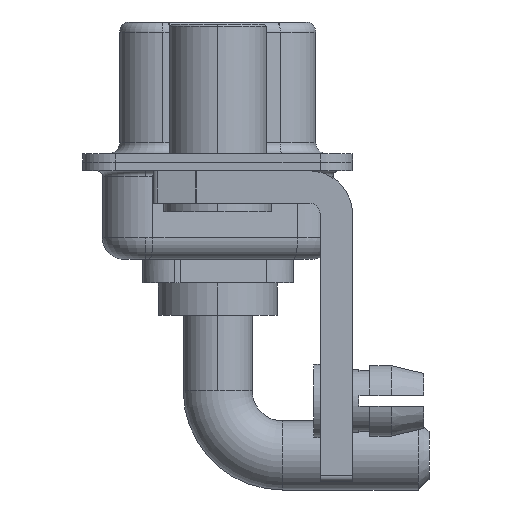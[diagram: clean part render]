
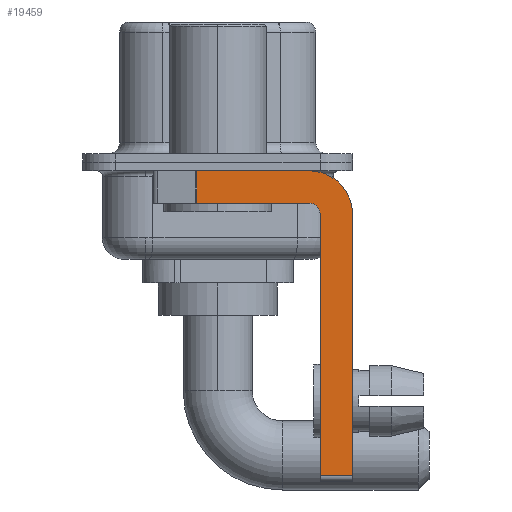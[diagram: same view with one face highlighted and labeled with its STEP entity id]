
A CAD part, left-side view. The second image highlights one B-rep face of the part: STEP entity #19459.
In plain terms, the highlighted planar face has unit normal (-1, 0, 0).
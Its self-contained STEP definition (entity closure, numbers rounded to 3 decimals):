
#223 = VERTEX_POINT ( 'NONE', #592 ) ;
#592 = CARTESIAN_POINT ( 'NONE',  ( -2.9, -6.25, -14.55 ) ) ;
#1279 = CARTESIAN_POINT ( 'NONE',  ( -2.9, -4.25, -14.55 ) ) ;
#1299 = VECTOR ( 'NONE', #8342, 1000. ) ;
#1378 = ORIENTED_EDGE ( 'NONE', *, *, #16896, .F. ) ;
#1668 = VERTEX_POINT ( 'NONE', #7297 ) ;
#1797 = CIRCLE ( 'NONE', #13898, 0.5 ) ;
#2083 = LINE ( 'NONE', #5151, #1299 ) ;
#2265 = CIRCLE ( 'NONE', #13045, 2. ) ;
#2371 = CARTESIAN_POINT ( 'NONE',  ( -2.9, -4.75, -14.8 ) ) ;
#2719 = VERTEX_POINT ( 'NONE', #2897 ) ;
#2897 = CARTESIAN_POINT ( 'NONE',  ( -2.9, -4.75, -2.4 ) ) ;
#2933 = EDGE_CURVE ( 'NONE', #13169, #2719, #6983, .T. ) ;
#3013 = CARTESIAN_POINT ( 'NONE',  ( -2.9, -4.25, -2.4 ) ) ;
#3031 = VERTEX_POINT ( 'NONE', #8624 ) ;
#3489 = EDGE_LOOP ( 'NONE', ( #1378, #7962, #15100, #5700, #3946, #11951, #7807, #8124 ) ) ;
#3511 = LINE ( 'NONE', #18599, #12424 ) ;
#3946 = ORIENTED_EDGE ( 'NONE', *, *, #2933, .F. ) ;
#4047 = VERTEX_POINT ( 'NONE', #20202 ) ;
#4149 = DIRECTION ( 'NONE',  ( 0., -1., 0. ) ) ;
#4227 = DIRECTION ( 'NONE',  ( -1., 0., 0. ) ) ;
#4255 = LINE ( 'NONE', #1279, #16147 ) ;
#4931 = VECTOR ( 'NONE', #8216, 1000. ) ;
#5151 = CARTESIAN_POINT ( 'NONE',  ( -2.9, 0.978, -1.9 ) ) ;
#5385 = EDGE_CURVE ( 'NONE', #1668, #9823, #2265, .T. ) ;
#5649 = CARTESIAN_POINT ( 'NONE',  ( -2.9, -4.25, -2.4 ) ) ;
#5700 = ORIENTED_EDGE ( 'NONE', *, *, #12067, .F. ) ;
#6328 = LINE ( 'NONE', #7875, #10740 ) ;
#6983 = LINE ( 'NONE', #2371, #4931 ) ;
#7297 = CARTESIAN_POINT ( 'NONE',  ( -2.9, -4.25, -0.4 ) ) ;
#7553 = CARTESIAN_POINT ( 'NONE',  ( -2.9, -4.75, -14.55 ) ) ;
#7807 = ORIENTED_EDGE ( 'NONE', *, *, #20039, .F. ) ;
#7875 = CARTESIAN_POINT ( 'NONE',  ( -2.9, -4.25, -1.9 ) ) ;
#7962 = ORIENTED_EDGE ( 'NONE', *, *, #10105, .T. ) ;
#8124 = ORIENTED_EDGE ( 'NONE', *, *, #5385, .F. ) ;
#8216 = DIRECTION ( 'NONE',  ( 0., 0., 1. ) ) ;
#8342 = DIRECTION ( 'NONE',  ( 0., 0., -1. ) ) ;
#8624 = CARTESIAN_POINT ( 'NONE',  ( -2.9, -4.25, -1.9 ) ) ;
#9043 = CARTESIAN_POINT ( 'NONE',  ( -2.9, -4.25, -2.4 ) ) ;
#9421 = DIRECTION ( 'NONE',  ( 1., 0., 0. ) ) ;
#9756 = DIRECTION ( 'NONE',  ( 0., 0., -1. ) ) ;
#9823 = VERTEX_POINT ( 'NONE', #13575 ) ;
#10105 = EDGE_CURVE ( 'NONE', #10445, #4047, #2083, .T. ) ;
#10445 = VERTEX_POINT ( 'NONE', #19440 ) ;
#10740 = VECTOR ( 'NONE', #17358, 1000. ) ;
#10761 = PLANE ( 'NONE',  #12392 ) ;
#11538 = LINE ( 'NONE', #18067, #13856 ) ;
#11951 = ORIENTED_EDGE ( 'NONE', *, *, #17149, .T. ) ;
#12067 = EDGE_CURVE ( 'NONE', #2719, #3031, #1797, .T. ) ;
#12236 = DIRECTION ( 'NONE',  ( 1., 0., 0. ) ) ;
#12392 = AXIS2_PLACEMENT_3D ( 'NONE', #5649, #9421, #14307 ) ;
#12424 = VECTOR ( 'NONE', #9756, 1000. ) ;
#13045 = AXIS2_PLACEMENT_3D ( 'NONE', #3013, #12236, #13768 ) ;
#13169 = VERTEX_POINT ( 'NONE', #7553 ) ;
#13575 = CARTESIAN_POINT ( 'NONE',  ( -2.9, -6.25, -2.4 ) ) ;
#13768 = DIRECTION ( 'NONE',  ( 0., 0., -1. ) ) ;
#13856 = VECTOR ( 'NONE', #14568, 1000. ) ;
#13898 = AXIS2_PLACEMENT_3D ( 'NONE', #9043, #4227, #16714 ) ;
#14307 = DIRECTION ( 'NONE',  ( 0., 0., -1. ) ) ;
#14568 = DIRECTION ( 'NONE',  ( 0., -1., 0. ) ) ;
#15100 = ORIENTED_EDGE ( 'NONE', *, *, #18198, .F. ) ;
#16147 = VECTOR ( 'NONE', #4149, 1000. ) ;
#16714 = DIRECTION ( 'NONE',  ( 0., 0., 1. ) ) ;
#16896 = EDGE_CURVE ( 'NONE', #10445, #1668, #11538, .T. ) ;
#17149 = EDGE_CURVE ( 'NONE', #13169, #223, #4255, .T. ) ;
#17358 = DIRECTION ( 'NONE',  ( 0., 1., 0. ) ) ;
#18067 = CARTESIAN_POINT ( 'NONE',  ( -2.9, 3., -0.4 ) ) ;
#18198 = EDGE_CURVE ( 'NONE', #3031, #4047, #6328, .T. ) ;
#18599 = CARTESIAN_POINT ( 'NONE',  ( -2.9, -6.25, -2.4 ) ) ;
#19440 = CARTESIAN_POINT ( 'NONE',  ( -2.9, 0.978, -0.4 ) ) ;
#19459 = ADVANCED_FACE ( 'NONE', ( #20074 ), #10761, .F. ) ;
#20039 = EDGE_CURVE ( 'NONE', #9823, #223, #3511, .T. ) ;
#20074 = FACE_OUTER_BOUND ( 'NONE', #3489, .T. ) ;
#20202 = CARTESIAN_POINT ( 'NONE',  ( -2.9, 0.978, -1.9 ) ) ;
